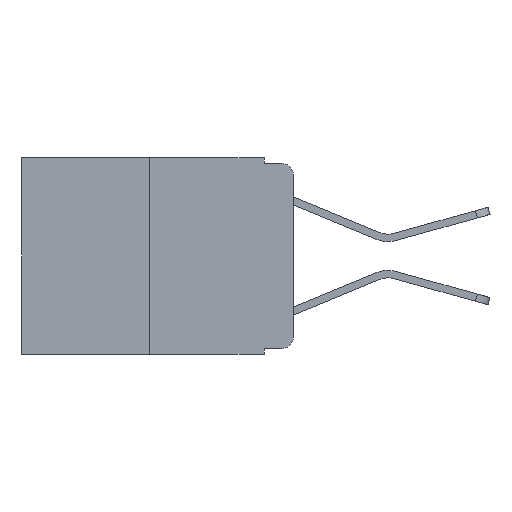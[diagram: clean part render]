
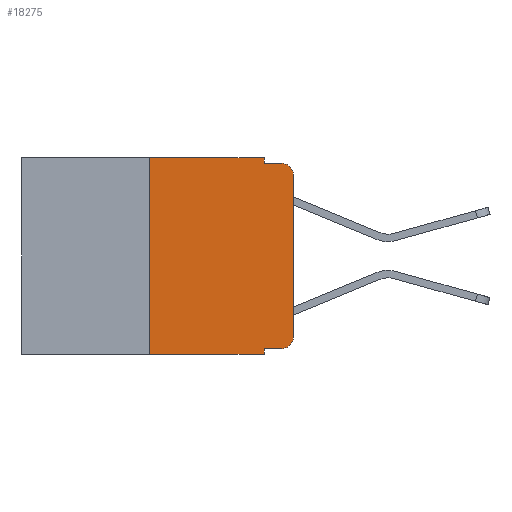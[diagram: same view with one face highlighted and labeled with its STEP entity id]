
A CAD part, left-side view. The second image highlights one B-rep face of the part: STEP entity #18275.
In plain terms, the highlighted planar face has unit normal (-1, 0, 0).
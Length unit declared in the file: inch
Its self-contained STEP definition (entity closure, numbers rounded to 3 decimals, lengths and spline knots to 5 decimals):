
#578 = EDGE_LOOP ( 'NONE', ( #19607, #12628, #12884, #1906, #698, #4576, #8180, #13688, #727, #7994 ) ) ;
#698 = ORIENTED_EDGE ( 'NONE', *, *, #21026, .F. ) ;
#727 = ORIENTED_EDGE ( 'NONE', *, *, #8689, .T. ) ;
#1021 = VERTEX_POINT ( 'NONE', #8344 ) ;
#1265 = LINE ( 'NONE', #9440, #13552 ) ;
#1381 = LINE ( 'NONE', #7209, #17073 ) ;
#1655 = VERTEX_POINT ( 'NONE', #7233 ) ;
#1858 = DIRECTION ( 'NONE',  ( 0., 0., -1. ) ) ;
#1906 = ORIENTED_EDGE ( 'NONE', *, *, #2156, .F. ) ;
#2156 = EDGE_CURVE ( 'NONE', #16564, #19790, #6185, .T. ) ;
#2466 = CARTESIAN_POINT ( 'NONE',  ( 0., 0.051, -0.333 ) ) ;
#2705 = VERTEX_POINT ( 'NONE', #20810 ) ;
#2848 = LINE ( 'NONE', #22006, #13168 ) ;
#4017 = CARTESIAN_POINT ( 'NONE',  ( 0., 0.25, 0. ) ) ;
#4576 = ORIENTED_EDGE ( 'NONE', *, *, #19022, .F. ) ;
#4816 = CIRCLE ( 'NONE', #16106, 0.02 ) ;
#4932 = LINE ( 'NONE', #7879, #24909 ) ;
#5026 = VERTEX_POINT ( 'NONE', #13150 ) ;
#5147 = DIRECTION ( 'NONE',  ( 0., 0., 1. ) ) ;
#6185 = LINE ( 'NONE', #22261, #21612 ) ;
#6360 = CARTESIAN_POINT ( 'NONE',  ( 0., 0.02, -0.333 ) ) ;
#7209 = CARTESIAN_POINT ( 'NONE',  ( 0., 0.051, -0.01 ) ) ;
#7233 = CARTESIAN_POINT ( 'NONE',  ( 0., 0., -0.313 ) ) ;
#7879 = CARTESIAN_POINT ( 'NONE',  ( 0., 0.473, 0. ) ) ;
#7994 = ORIENTED_EDGE ( 'NONE', *, *, #21308, .T. ) ;
#8147 = CARTESIAN_POINT ( 'NONE',  ( 0., 0.02, -0.03 ) ) ;
#8180 = ORIENTED_EDGE ( 'NONE', *, *, #22602, .T. ) ;
#8291 = DIRECTION ( 'NONE',  ( 0., 0., -1. ) ) ;
#8344 = CARTESIAN_POINT ( 'NONE',  ( 0., 0., -0.03 ) ) ;
#8689 = EDGE_CURVE ( 'NONE', #5026, #21692, #19151, .T. ) ;
#8835 = VERTEX_POINT ( 'NONE', #21037 ) ;
#8846 = FACE_OUTER_BOUND ( 'NONE', #578, .T. ) ;
#9209 = VERTEX_POINT ( 'NONE', #16236 ) ;
#9440 = CARTESIAN_POINT ( 'NONE',  ( 0., 0.473, -0.343 ) ) ;
#10003 = CARTESIAN_POINT ( 'NONE',  ( 0., 0.051, 0. ) ) ;
#10066 = EDGE_CURVE ( 'NONE', #5026, #2705, #2848, .T. ) ;
#10205 = DIRECTION ( 'NONE',  ( 0., 0., -1. ) ) ;
#10653 = DIRECTION ( 'NONE',  ( 0., -1., 0. ) ) ;
#10866 = CARTESIAN_POINT ( 'NONE',  ( 0., 0.02, -0.313 ) ) ;
#11386 = LINE ( 'NONE', #21302, #16155 ) ;
#11432 = DIRECTION ( 'NONE',  ( 0., 0., -1. ) ) ;
#12628 = ORIENTED_EDGE ( 'NONE', *, *, #14576, .T. ) ;
#12641 = VECTOR ( 'NONE', #10653, 39.37008 ) ;
#12884 = ORIENTED_EDGE ( 'NONE', *, *, #13217, .F. ) ;
#12969 = DIRECTION ( 'NONE',  ( 0., 0., -1. ) ) ;
#13150 = CARTESIAN_POINT ( 'NONE',  ( 0., 0.051, -0.333 ) ) ;
#13168 = VECTOR ( 'NONE', #1858, 39.37008 ) ;
#13217 = EDGE_CURVE ( 'NONE', #19790, #9209, #1381, .T. ) ;
#13444 = CARTESIAN_POINT ( 'NONE',  ( 0., 0.473, 0. ) ) ;
#13552 = VECTOR ( 'NONE', #21447, 39.37008 ) ;
#13688 = ORIENTED_EDGE ( 'NONE', *, *, #10066, .F. ) ;
#14576 = EDGE_CURVE ( 'NONE', #1021, #9209, #4816, .T. ) ;
#14722 = VECTOR ( 'NONE', #25876, 39.37008 ) ;
#15353 = LINE ( 'NONE', #23960, #14722 ) ;
#15451 = PLANE ( 'NONE',  #20747 ) ;
#15789 = CARTESIAN_POINT ( 'NONE',  ( 0., 0.051, -0.01 ) ) ;
#16010 = DIRECTION ( 'NONE',  ( 0., -1., 0. ) ) ;
#16106 = AXIS2_PLACEMENT_3D ( 'NONE', #8147, #22153, #10205 ) ;
#16155 = VECTOR ( 'NONE', #5147, 39.37008 ) ;
#16236 = CARTESIAN_POINT ( 'NONE',  ( 0., 0.02, -0.01 ) ) ;
#16564 = VERTEX_POINT ( 'NONE', #10003 ) ;
#17073 = VECTOR ( 'NONE', #21285, 39.37008 ) ;
#18275 = ADVANCED_FACE ( 'NONE', ( #8846 ), #15451, .F. ) ;
#18882 = CIRCLE ( 'NONE', #24956, 0.02 ) ;
#19022 = EDGE_CURVE ( 'NONE', #8835, #24392, #11386, .T. ) ;
#19151 = LINE ( 'NONE', #2466, #12641 ) ;
#19607 = ORIENTED_EDGE ( 'NONE', *, *, #24987, .T. ) ;
#19790 = VERTEX_POINT ( 'NONE', #15789 ) ;
#20747 = AXIS2_PLACEMENT_3D ( 'NONE', #13444, #23247, #11432 ) ;
#20810 = CARTESIAN_POINT ( 'NONE',  ( 0., 0.051, -0.343 ) ) ;
#21026 = EDGE_CURVE ( 'NONE', #24392, #16564, #4932, .T. ) ;
#21037 = CARTESIAN_POINT ( 'NONE',  ( 0., 0.25, -0.343 ) ) ;
#21285 = DIRECTION ( 'NONE',  ( 0., -1., 0. ) ) ;
#21302 = CARTESIAN_POINT ( 'NONE',  ( 0., 0.25, 0. ) ) ;
#21308 = EDGE_CURVE ( 'NONE', #21692, #1655, #18882, .T. ) ;
#21447 = DIRECTION ( 'NONE',  ( 0., -1., 0. ) ) ;
#21612 = VECTOR ( 'NONE', #8291, 39.37008 ) ;
#21692 = VERTEX_POINT ( 'NONE', #6360 ) ;
#22006 = CARTESIAN_POINT ( 'NONE',  ( 0., 0.051, 0. ) ) ;
#22153 = DIRECTION ( 'NONE',  ( -1., 0., 0. ) ) ;
#22261 = CARTESIAN_POINT ( 'NONE',  ( 0., 0.051, 0. ) ) ;
#22602 = EDGE_CURVE ( 'NONE', #8835, #2705, #1265, .T. ) ;
#23247 = DIRECTION ( 'NONE',  ( 1., 0., 0. ) ) ;
#23960 = CARTESIAN_POINT ( 'NONE',  ( 0., 0., 0. ) ) ;
#24392 = VERTEX_POINT ( 'NONE', #4017 ) ;
#24671 = DIRECTION ( 'NONE',  ( -1., 0., 0. ) ) ;
#24909 = VECTOR ( 'NONE', #16010, 39.37008 ) ;
#24956 = AXIS2_PLACEMENT_3D ( 'NONE', #10866, #24671, #12969 ) ;
#24987 = EDGE_CURVE ( 'NONE', #1655, #1021, #15353, .T. ) ;
#25876 = DIRECTION ( 'NONE',  ( 0., 0., 1. ) ) ;
